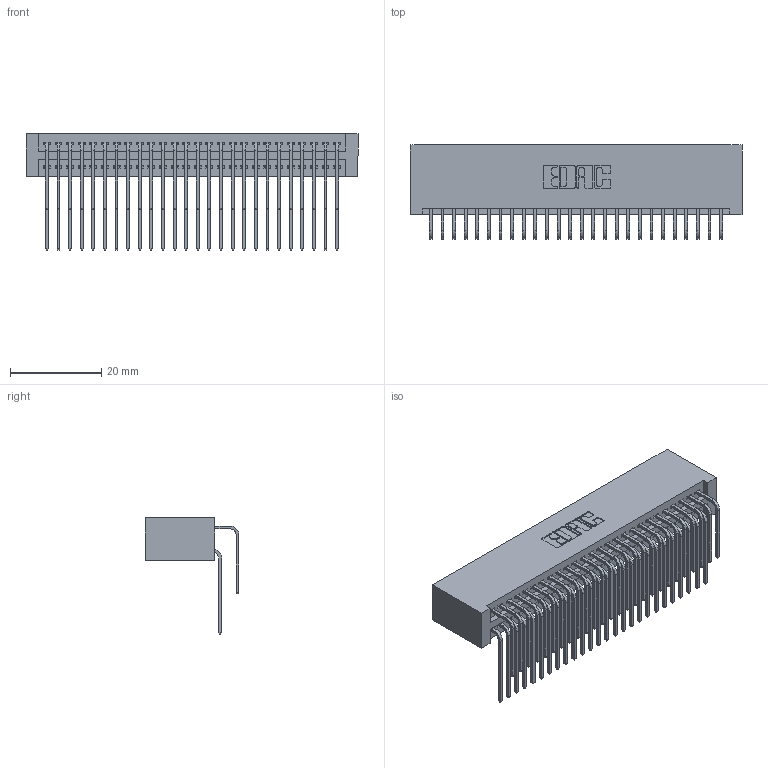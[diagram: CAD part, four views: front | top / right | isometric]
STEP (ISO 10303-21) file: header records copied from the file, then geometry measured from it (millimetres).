
FILE_DESCRIPTION (( 'STEP AP203' ), '1' );
FILE_NAME ('395-052-559-201.STEP', '2019-10-19T15:56:06', ( '' ), ( '' ), 'SwSTEP 2.0', 'SolidWorks 2016', '' );
FILE_SCHEMA (( 'CONFIG_CONTROL_DESIGN' ));
Length unit declared in the file: inch
Products named in the file (4): 345 Part_No Mounting Lugs; 345-292-001_558 559 Tail - 1; 345-292-001_559 Tail - 2; 395-052-559-201
Assembly tree (53 placements, depth 2):
  395-052-559-201
    345 Part_No Mounting Lugs
    345-292-001_558 559 Tail - 1  x26
    345-292-001_559 Tail - 2  x26
Bounding box: 72.64 x 20.56 x 25.53 mm (x, y, z)
Volume: 7824.1 mm3; surface area: 12969.3 mm2
Topology: 53 solids, 53 shells, 2822 faces, 8377 edges, 5514 vertices
Faces by surface type: plane 1896, cylinder 926
Entity records: 23929 total; most frequent: CARTESIAN_POINT 4071, ORIENTED_EDGE 3954, DIRECTION 3577, EDGE_CURVE 1977, VECTOR 1709, LINE 1709, VERTEX_POINT 1314, AXIS2_PLACEMENT_3D 934
